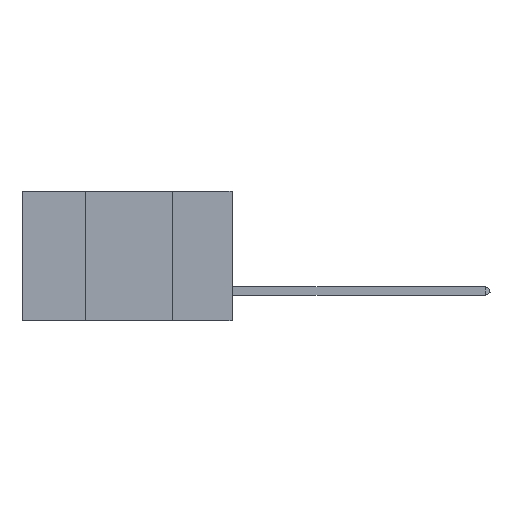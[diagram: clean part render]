
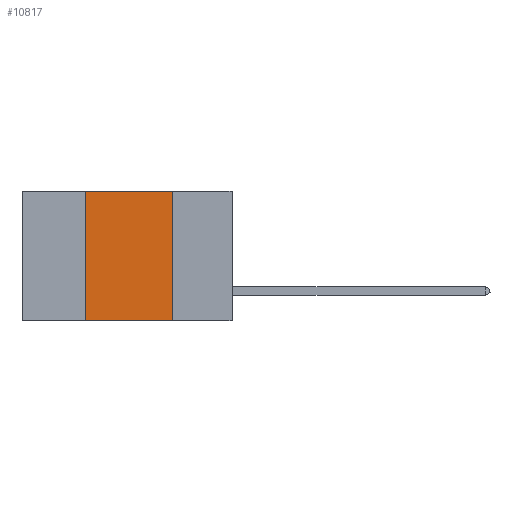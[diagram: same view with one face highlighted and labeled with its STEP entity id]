
A CAD part, left-side view. The second image highlights one B-rep face of the part: STEP entity #10817.
In plain terms, the highlighted planar face has unit normal (-1, 0, 0).
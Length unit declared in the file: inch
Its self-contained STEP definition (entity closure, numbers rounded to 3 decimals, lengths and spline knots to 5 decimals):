
#509 = CARTESIAN_POINT ( 'NONE',  ( 0., 0.42, 0. ) ) ;
#1026 = EDGE_CURVE ( 'NONE', #20891, #35049, #28684, .T. ) ;
#3326 = ORIENTED_EDGE ( 'NONE', *, *, #25234, .T. ) ;
#5964 = DIRECTION ( 'NONE',  ( 0., 0., -1. ) ) ;
#7568 = VECTOR ( 'NONE', #20895, 39.37008 ) ;
#8308 = EDGE_CURVE ( 'NONE', #40566, #10368, #27357, .T. ) ;
#10368 = VERTEX_POINT ( 'NONE', #42220 ) ;
#10817 = ADVANCED_FACE ( 'NONE', ( #40246 ), #35925, .F. ) ;
#11122 = LINE ( 'NONE', #13863, #11686 ) ;
#11686 = VECTOR ( 'NONE', #24516, 39.37008 ) ;
#13863 = CARTESIAN_POINT ( 'NONE',  ( 0., 0.6, 0. ) ) ;
#15296 = DIRECTION ( 'NONE',  ( 0., 0., -1. ) ) ;
#18554 = VECTOR ( 'NONE', #42649, 39.37008 ) ;
#20891 = VERTEX_POINT ( 'NONE', #40714 ) ;
#20895 = DIRECTION ( 'NONE',  ( 0., -1., 0. ) ) ;
#24516 = DIRECTION ( 'NONE',  ( 0., -1., 0. ) ) ;
#24792 = AXIS2_PLACEMENT_3D ( 'NONE', #29077, #36071, #15296 ) ;
#25234 = EDGE_CURVE ( 'NONE', #20891, #10368, #36251, .T. ) ;
#25543 = ORIENTED_EDGE ( 'NONE', *, *, #1026, .F. ) ;
#25930 = CARTESIAN_POINT ( 'NONE',  ( 0., 0.42, 0. ) ) ;
#27357 = LINE ( 'NONE', #36116, #33254 ) ;
#28684 = LINE ( 'NONE', #25930, #18554 ) ;
#29077 = CARTESIAN_POINT ( 'NONE',  ( 0., 0.6, 0. ) ) ;
#29324 = EDGE_LOOP ( 'NONE', ( #35929, #39427, #25543, #3326 ) ) ;
#31788 = CARTESIAN_POINT ( 'NONE',  ( 0., 0.6, -0.37 ) ) ;
#33254 = VECTOR ( 'NONE', #5964, 39.37008 ) ;
#34752 = CARTESIAN_POINT ( 'NONE',  ( 0., 0.17, 0. ) ) ;
#35049 = VERTEX_POINT ( 'NONE', #509 ) ;
#35925 = PLANE ( 'NONE',  #24792 ) ;
#35929 = ORIENTED_EDGE ( 'NONE', *, *, #8308, .F. ) ;
#36071 = DIRECTION ( 'NONE',  ( 1., 0., 0. ) ) ;
#36116 = CARTESIAN_POINT ( 'NONE',  ( 0., 0.17, 0. ) ) ;
#36251 = LINE ( 'NONE', #31788, #7568 ) ;
#37036 = EDGE_CURVE ( 'NONE', #35049, #40566, #11122, .T. ) ;
#39427 = ORIENTED_EDGE ( 'NONE', *, *, #37036, .F. ) ;
#40246 = FACE_OUTER_BOUND ( 'NONE', #29324, .T. ) ;
#40566 = VERTEX_POINT ( 'NONE', #34752 ) ;
#40714 = CARTESIAN_POINT ( 'NONE',  ( 0., 0.42, -0.37 ) ) ;
#42220 = CARTESIAN_POINT ( 'NONE',  ( 0., 0.17, -0.37 ) ) ;
#42649 = DIRECTION ( 'NONE',  ( 0., 0., 1. ) ) ;
